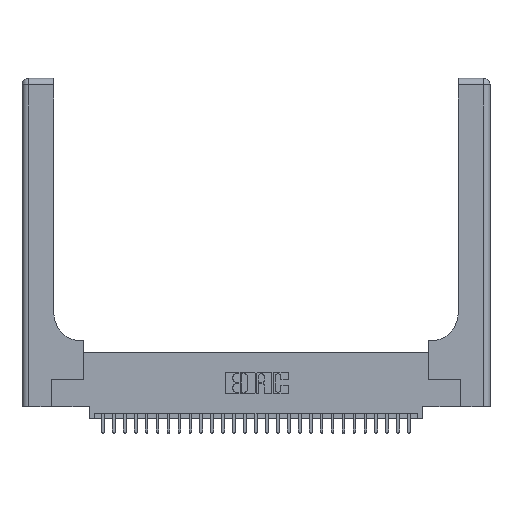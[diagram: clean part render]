
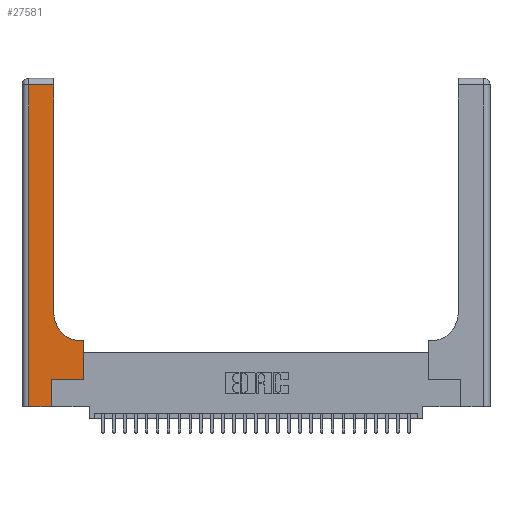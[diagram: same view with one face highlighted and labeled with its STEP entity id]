
A CAD part, top view. The second image highlights one B-rep face of the part: STEP entity #27581.
In plain terms, the highlighted planar face has unit normal (0, 0, 1).
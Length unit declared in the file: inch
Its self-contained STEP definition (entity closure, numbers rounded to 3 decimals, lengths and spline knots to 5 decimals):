
#410 = LINE ( 'NONE', #8902, #5868 ) ;
#1211 = VECTOR ( 'NONE', #5785, 39.37008 ) ;
#2003 = CARTESIAN_POINT ( 'NONE',  ( 0.269, 0., 0.37 ) ) ;
#2253 = LINE ( 'NONE', #21075, #6996 ) ;
#2728 = PLANE ( 'NONE',  #13688 ) ;
#3280 = CARTESIAN_POINT ( 'NONE',  ( 0.5585, 0.25, 0.37 ) ) ;
#3583 = LINE ( 'NONE', #26621, #26695 ) ;
#3888 = EDGE_CURVE ( 'NONE', #5134, #29847, #410, .T. ) ;
#4701 = CARTESIAN_POINT ( 'NONE',  ( 0.2915, 0.85, 0.37 ) ) ;
#4900 = CARTESIAN_POINT ( 'NONE',  ( 0.5585, 0.25, 0.37 ) ) ;
#5081 = DIRECTION ( 'NONE',  ( 0., 0., -1. ) ) ;
#5134 = VERTEX_POINT ( 'NONE', #29198 ) ;
#5347 = LINE ( 'NONE', #27667, #23092 ) ;
#5575 = ORIENTED_EDGE ( 'NONE', *, *, #16192, .T. ) ;
#5674 = LINE ( 'NONE', #4900, #23406 ) ;
#5785 = DIRECTION ( 'NONE',  ( 0., -1., 0. ) ) ;
#5868 = VECTOR ( 'NONE', #22743, 39.37008 ) ;
#6460 = EDGE_CURVE ( 'NONE', #24801, #22027, #5347, .T. ) ;
#6996 = VECTOR ( 'NONE', #11884, 39.37008 ) ;
#7040 = ORIENTED_EDGE ( 'NONE', *, *, #17546, .T. ) ;
#7236 = DIRECTION ( 'NONE',  ( 0., 1., 0. ) ) ;
#7369 = ORIENTED_EDGE ( 'NONE', *, *, #9295, .T. ) ;
#7432 = VERTEX_POINT ( 'NONE', #28967 ) ;
#8482 = CARTESIAN_POINT ( 'NONE',  ( 0., 2.94, 0.37 ) ) ;
#8892 = VERTEX_POINT ( 'NONE', #22506 ) ;
#8902 = CARTESIAN_POINT ( 'NONE',  ( 0., 0., 0.37 ) ) ;
#9295 = EDGE_CURVE ( 'NONE', #8892, #5134, #13597, .T. ) ;
#9932 = ORIENTED_EDGE ( 'NONE', *, *, #24749, .T. ) ;
#11153 = CARTESIAN_POINT ( 'NONE',  ( 0.5585, 0.6, 0.37 ) ) ;
#11884 = DIRECTION ( 'NONE',  ( -1., 0., 0. ) ) ;
#11933 = EDGE_LOOP ( 'NONE', ( #9932, #29639, #7369, #15043, #21158, #28599, #5575, #7040, #13234 ) ) ;
#12108 = DIRECTION ( 'NONE',  ( 1., 0., 0. ) ) ;
#12302 = CARTESIAN_POINT ( 'NONE',  ( 0.5415, 0.85, 0.37 ) ) ;
#12470 = FACE_OUTER_BOUND ( 'NONE', #11933, .T. ) ;
#12617 = CIRCLE ( 'NONE', #22420, 0.25 ) ;
#13234 = ORIENTED_EDGE ( 'NONE', *, *, #14947, .T. ) ;
#13274 = DIRECTION ( 'NONE',  ( -1., 0., 0. ) ) ;
#13597 = LINE ( 'NONE', #19687, #1211 ) ;
#13656 = EDGE_CURVE ( 'NONE', #29847, #24801, #3583, .T. ) ;
#13688 = AXIS2_PLACEMENT_3D ( 'NONE', #23503, #5081, #21299 ) ;
#14646 = DIRECTION ( 'NONE',  ( 1., 0., 0. ) ) ;
#14947 = EDGE_CURVE ( 'NONE', #28186, #16118, #12617, .T. ) ;
#15043 = ORIENTED_EDGE ( 'NONE', *, *, #3888, .T. ) ;
#15929 = EDGE_CURVE ( 'NONE', #7432, #8892, #24492, .T. ) ;
#16118 = VERTEX_POINT ( 'NONE', #4701 ) ;
#16192 = EDGE_CURVE ( 'NONE', #22027, #21653, #5674, .T. ) ;
#16751 = CARTESIAN_POINT ( 'NONE',  ( 0.5415, 0.6, 0.37 ) ) ;
#17546 = EDGE_CURVE ( 'NONE', #21653, #28186, #2253, .T. ) ;
#18074 = VECTOR ( 'NONE', #28982, 39.37008 ) ;
#18404 = VECTOR ( 'NONE', #13274, 39.37008 ) ;
#19687 = CARTESIAN_POINT ( 'NONE',  ( 0.06, 3., 0.37 ) ) ;
#20342 = CARTESIAN_POINT ( 'NONE',  ( 0.269, 0.25, 0.37 ) ) ;
#21075 = CARTESIAN_POINT ( 'NONE',  ( 0.2915, 0.6, 0.37 ) ) ;
#21158 = ORIENTED_EDGE ( 'NONE', *, *, #13656, .T. ) ;
#21299 = DIRECTION ( 'NONE',  ( -1., 0., 0. ) ) ;
#21653 = VERTEX_POINT ( 'NONE', #11153 ) ;
#22027 = VERTEX_POINT ( 'NONE', #3280 ) ;
#22420 = AXIS2_PLACEMENT_3D ( 'NONE', #12302, #28316, #14646 ) ;
#22506 = CARTESIAN_POINT ( 'NONE',  ( 0.06, 2.94, 0.37 ) ) ;
#22743 = DIRECTION ( 'NONE',  ( 1., 0., 0. ) ) ;
#23092 = VECTOR ( 'NONE', #12108, 39.37008 ) ;
#23406 = VECTOR ( 'NONE', #7236, 39.37008 ) ;
#23503 = CARTESIAN_POINT ( 'NONE',  ( 0., 3., 0.37 ) ) ;
#24450 = DIRECTION ( 'NONE',  ( 0., 1., 0. ) ) ;
#24492 = LINE ( 'NONE', #8482, #18404 ) ;
#24749 = EDGE_CURVE ( 'NONE', #16118, #7432, #24881, .T. ) ;
#24801 = VERTEX_POINT ( 'NONE', #20342 ) ;
#24881 = LINE ( 'NONE', #26722, #18074 ) ;
#26621 = CARTESIAN_POINT ( 'NONE',  ( 0.269, 0., 0.37 ) ) ;
#26695 = VECTOR ( 'NONE', #24450, 39.37008 ) ;
#26722 = CARTESIAN_POINT ( 'NONE',  ( 0.2915, 3., 0.37 ) ) ;
#27581 = ADVANCED_FACE ( 'NONE', ( #12470 ), #2728, .F. ) ;
#27667 = CARTESIAN_POINT ( 'NONE',  ( 0.269, 0.25, 0.37 ) ) ;
#28186 = VERTEX_POINT ( 'NONE', #16751 ) ;
#28316 = DIRECTION ( 'NONE',  ( 0., 0., -1. ) ) ;
#28599 = ORIENTED_EDGE ( 'NONE', *, *, #6460, .T. ) ;
#28967 = CARTESIAN_POINT ( 'NONE',  ( 0.2915, 2.94, 0.37 ) ) ;
#28982 = DIRECTION ( 'NONE',  ( 0., 1., 0. ) ) ;
#29198 = CARTESIAN_POINT ( 'NONE',  ( 0.06, 0., 0.37 ) ) ;
#29639 = ORIENTED_EDGE ( 'NONE', *, *, #15929, .T. ) ;
#29847 = VERTEX_POINT ( 'NONE', #2003 ) ;
